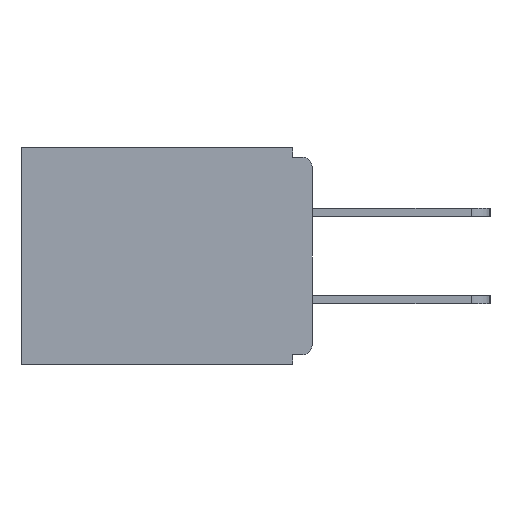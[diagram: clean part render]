
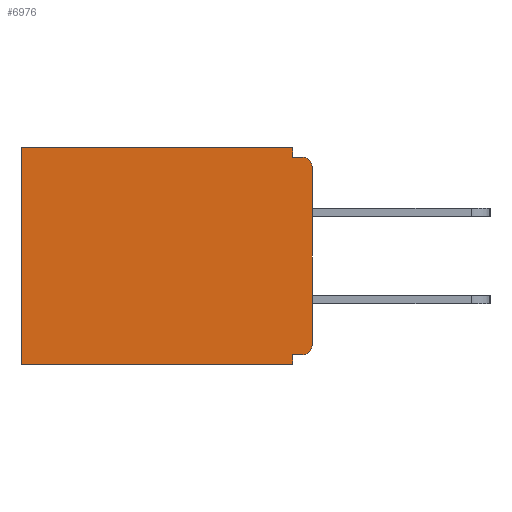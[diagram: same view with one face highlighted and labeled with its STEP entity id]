
A CAD part, left-side view. The second image highlights one B-rep face of the part: STEP entity #6976.
In plain terms, the highlighted planar face has unit normal (-1, 0, 0).
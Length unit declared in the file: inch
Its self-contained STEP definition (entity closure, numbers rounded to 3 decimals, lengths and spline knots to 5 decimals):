
#188 = CIRCLE ( 'NONE', #3980, 0.015 ) ;
#266 = DIRECTION ( 'NONE',  ( 0., 0., -1. ) ) ;
#309 = CARTESIAN_POINT ( 'NONE',  ( 0.298, 0.015, -0.328 ) ) ;
#492 = CARTESIAN_POINT ( 'NONE',  ( 0.298, 0.46, 0. ) ) ;
#699 = LINE ( 'NONE', #5575, #6805 ) ;
#965 = DIRECTION ( 'NONE',  ( 0., 0., -1. ) ) ;
#1175 = EDGE_LOOP ( 'NONE', ( #9538, #23884, #9272, #2763, #11133, #14699, #16139, #18556, #14352, #5541 ) ) ;
#1772 = DIRECTION ( 'NONE',  ( 0., 1., 0. ) ) ;
#1902 = EDGE_CURVE ( 'NONE', #14119, #14789, #4042, .T. ) ;
#1965 = CARTESIAN_POINT ( 'NONE',  ( 0.298, 0.031, 0. ) ) ;
#2289 = EDGE_CURVE ( 'NONE', #9009, #12924, #4019, .T. ) ;
#2763 = ORIENTED_EDGE ( 'NONE', *, *, #4974, .T. ) ;
#3002 = AXIS2_PLACEMENT_3D ( 'NONE', #21421, #10425, #4833 ) ;
#3092 = CARTESIAN_POINT ( 'NONE',  ( 0.298, 0.46, -0.343 ) ) ;
#3107 = DIRECTION ( 'NONE',  ( 0., 1., 0. ) ) ;
#3980 = AXIS2_PLACEMENT_3D ( 'NONE', #6756, #4899, #14172 ) ;
#4019 = LINE ( 'NONE', #19820, #23228 ) ;
#4042 = LINE ( 'NONE', #19958, #16250 ) ;
#4833 = DIRECTION ( 'NONE',  ( 0., 0., -1. ) ) ;
#4899 = DIRECTION ( 'NONE',  ( -1., 0., 0. ) ) ;
#4974 = EDGE_CURVE ( 'NONE', #7266, #6481, #13207, .T. ) ;
#5541 = ORIENTED_EDGE ( 'NONE', *, *, #18254, .F. ) ;
#5575 = CARTESIAN_POINT ( 'NONE',  ( 0.298, 0., -0.328 ) ) ;
#5640 = VECTOR ( 'NONE', #21074, 39.37008 ) ;
#5863 = VERTEX_POINT ( 'NONE', #9993 ) ;
#5885 = DIRECTION ( 'NONE',  ( 0., 1., 0. ) ) ;
#5946 = EDGE_CURVE ( 'NONE', #5863, #12924, #6470, .T. ) ;
#6470 = CIRCLE ( 'NONE', #13868, 0.015 ) ;
#6481 = VERTEX_POINT ( 'NONE', #23634 ) ;
#6756 = CARTESIAN_POINT ( 'NONE',  ( 0.298, 0.015, -0.313 ) ) ;
#6805 = VECTOR ( 'NONE', #1772, 39.37008 ) ;
#6821 = DIRECTION ( 'NONE',  ( -1., 0., 0. ) ) ;
#6976 = ADVANCED_FACE ( 'NONE', ( #9049 ), #12349, .F. ) ;
#6998 = VERTEX_POINT ( 'NONE', #10349 ) ;
#7266 = VERTEX_POINT ( 'NONE', #1965 ) ;
#7670 = VECTOR ( 'NONE', #5885, 39.37008 ) ;
#7686 = VECTOR ( 'NONE', #965, 39.37008 ) ;
#8005 = VECTOR ( 'NONE', #19183, 39.37008 ) ;
#8431 = CARTESIAN_POINT ( 'NONE',  ( 0.298, 0.031, -0.343 ) ) ;
#8459 = CARTESIAN_POINT ( 'NONE',  ( 0.298, 0.015, -0.03 ) ) ;
#8692 = CARTESIAN_POINT ( 'NONE',  ( 0.298, 0., 0. ) ) ;
#9009 = VERTEX_POINT ( 'NONE', #23007 ) ;
#9049 = FACE_OUTER_BOUND ( 'NONE', #1175, .T. ) ;
#9272 = ORIENTED_EDGE ( 'NONE', *, *, #18114, .F. ) ;
#9538 = ORIENTED_EDGE ( 'NONE', *, *, #5946, .T. ) ;
#9891 = CARTESIAN_POINT ( 'NONE',  ( 0.298, 0.031, -0.343 ) ) ;
#9993 = CARTESIAN_POINT ( 'NONE',  ( 0.298, 0., -0.03 ) ) ;
#10026 = LINE ( 'NONE', #8692, #7686 ) ;
#10168 = EDGE_CURVE ( 'NONE', #19752, #6998, #699, .T. ) ;
#10349 = CARTESIAN_POINT ( 'NONE',  ( 0.298, 0.031, -0.328 ) ) ;
#10425 = DIRECTION ( 'NONE',  ( 1., 0., 0. ) ) ;
#11133 = ORIENTED_EDGE ( 'NONE', *, *, #18570, .T. ) ;
#11602 = EDGE_CURVE ( 'NONE', #6998, #14119, #16312, .T. ) ;
#12349 = PLANE ( 'NONE',  #3002 ) ;
#12551 = DIRECTION ( 'NONE',  ( 0., -1., 0. ) ) ;
#12924 = VERTEX_POINT ( 'NONE', #16752 ) ;
#13207 = LINE ( 'NONE', #18822, #7670 ) ;
#13504 = LINE ( 'NONE', #492, #5640 ) ;
#13868 = AXIS2_PLACEMENT_3D ( 'NONE', #8459, #6821, #21482 ) ;
#14119 = VERTEX_POINT ( 'NONE', #8431 ) ;
#14172 = DIRECTION ( 'NONE',  ( 0., 0., -1. ) ) ;
#14352 = ORIENTED_EDGE ( 'NONE', *, *, #17129, .T. ) ;
#14699 = ORIENTED_EDGE ( 'NONE', *, *, #1902, .F. ) ;
#14789 = VERTEX_POINT ( 'NONE', #3092 ) ;
#15740 = VECTOR ( 'NONE', #266, 39.37008 ) ;
#16139 = ORIENTED_EDGE ( 'NONE', *, *, #11602, .F. ) ;
#16250 = VECTOR ( 'NONE', #3107, 39.37008 ) ;
#16312 = LINE ( 'NONE', #17150, #15740 ) ;
#16752 = CARTESIAN_POINT ( 'NONE',  ( 0.298, 0.015, -0.015 ) ) ;
#17129 = EDGE_CURVE ( 'NONE', #19752, #22024, #188, .T. ) ;
#17150 = CARTESIAN_POINT ( 'NONE',  ( 0.298, 0.031, -0.343 ) ) ;
#18114 = EDGE_CURVE ( 'NONE', #7266, #9009, #22838, .T. ) ;
#18254 = EDGE_CURVE ( 'NONE', #5863, #22024, #10026, .T. ) ;
#18556 = ORIENTED_EDGE ( 'NONE', *, *, #10168, .F. ) ;
#18570 = EDGE_CURVE ( 'NONE', #6481, #14789, #13504, .T. ) ;
#18822 = CARTESIAN_POINT ( 'NONE',  ( 0.298, 0., 0. ) ) ;
#19183 = DIRECTION ( 'NONE',  ( 0., 0., -1. ) ) ;
#19752 = VERTEX_POINT ( 'NONE', #309 ) ;
#19776 = CARTESIAN_POINT ( 'NONE',  ( 0.298, 0., -0.313 ) ) ;
#19820 = CARTESIAN_POINT ( 'NONE',  ( 0.298, 0., -0.015 ) ) ;
#19958 = CARTESIAN_POINT ( 'NONE',  ( 0.298, 0., -0.343 ) ) ;
#21074 = DIRECTION ( 'NONE',  ( 0., 0., -1. ) ) ;
#21421 = CARTESIAN_POINT ( 'NONE',  ( 0.298, 0., 0. ) ) ;
#21482 = DIRECTION ( 'NONE',  ( 0., 0., -1. ) ) ;
#22024 = VERTEX_POINT ( 'NONE', #19776 ) ;
#22838 = LINE ( 'NONE', #9891, #8005 ) ;
#23007 = CARTESIAN_POINT ( 'NONE',  ( 0.298, 0.031, -0.015 ) ) ;
#23228 = VECTOR ( 'NONE', #12551, 39.37008 ) ;
#23634 = CARTESIAN_POINT ( 'NONE',  ( 0.298, 0.46, 0. ) ) ;
#23884 = ORIENTED_EDGE ( 'NONE', *, *, #2289, .F. ) ;
